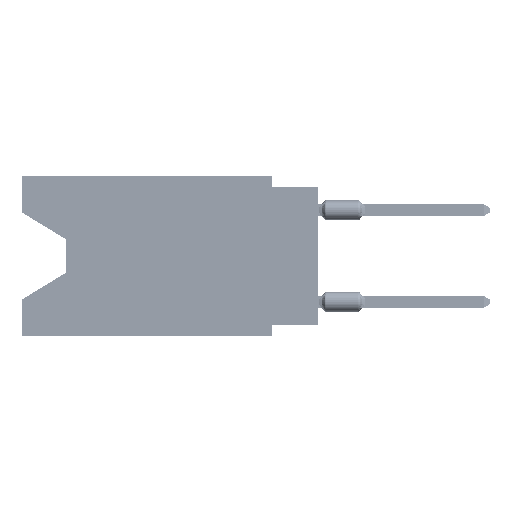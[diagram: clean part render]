
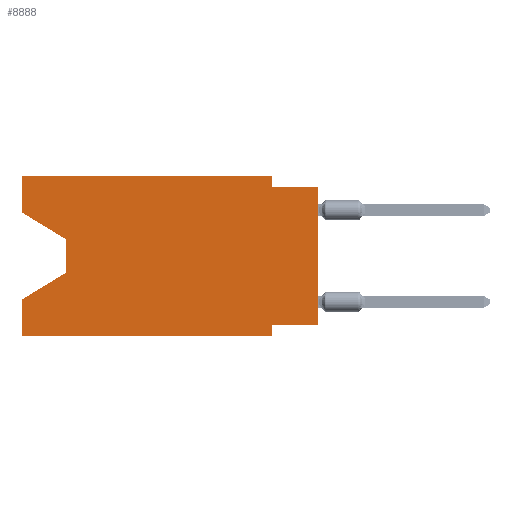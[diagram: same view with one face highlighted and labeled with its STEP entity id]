
A CAD part, left-side view. The second image highlights one B-rep face of the part: STEP entity #8888.
In plain terms, the highlighted planar face has unit normal (-1, 0, 0).
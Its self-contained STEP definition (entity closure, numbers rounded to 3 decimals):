
#288 = LINE ( 'NONE', #77231, #19993 ) ;
#1683 = LINE ( 'NONE', #27493, #95369 ) ;
#2556 = DIRECTION ( 'NONE',  ( 0., 0., -1. ) ) ;
#2775 = FACE_OUTER_BOUND ( 'NONE', #65414, .T. ) ;
#5400 = LINE ( 'NONE', #40770, #51607 ) ;
#8888 = ADVANCED_FACE ( 'NONE', ( #2775 ), #20752, .F. ) ;
#9208 = EDGE_CURVE ( 'NONE', #75606, #36875, #27916, .T. ) ;
#9214 = ORIENTED_EDGE ( 'NONE', *, *, #74387, .F. ) ;
#10415 = LINE ( 'NONE', #87878, #76460 ) ;
#10650 = DIRECTION ( 'NONE',  ( 0., 0.855, -0.519 ) ) ;
#13079 = ORIENTED_EDGE ( 'NONE', *, *, #45619, .F. ) ;
#13785 = EDGE_CURVE ( 'NONE', #82977, #32922, #1683, .T. ) ;
#15249 = VERTEX_POINT ( 'NONE', #76279 ) ;
#15433 = VECTOR ( 'NONE', #10650, 1000. ) ;
#15911 = LINE ( 'NONE', #50157, #105549 ) ;
#19244 = EDGE_CURVE ( 'NONE', #72556, #80418, #110894, .T. ) ;
#19993 = VECTOR ( 'NONE', #67709, 1000. ) ;
#20187 = DIRECTION ( 'NONE',  ( 0., 0., -1. ) ) ;
#20752 = PLANE ( 'NONE',  #31515 ) ;
#20849 = CARTESIAN_POINT ( 'NONE',  ( 0., 2.54, -0.635 ) ) ;
#22002 = VERTEX_POINT ( 'NONE', #46269 ) ;
#25535 = ORIENTED_EDGE ( 'NONE', *, *, #9208, .T. ) ;
#25588 = DIRECTION ( 'NONE',  ( 0., 0., 1. ) ) ;
#27133 = EDGE_CURVE ( 'NONE', #72268, #80418, #10415, .T. ) ;
#27493 = CARTESIAN_POINT ( 'NONE',  ( 0., 16.383, 0. ) ) ;
#27916 = LINE ( 'NONE', #103693, #65675 ) ;
#28185 = VECTOR ( 'NONE', #76021, 1000. ) ;
#28378 = DIRECTION ( 'NONE',  ( 0., -1., 0. ) ) ;
#29636 = EDGE_CURVE ( 'NONE', #94697, #36875, #5400, .T. ) ;
#30565 = CARTESIAN_POINT ( 'NONE',  ( 0., 16.383, -6.852 ) ) ;
#31515 = AXIS2_PLACEMENT_3D ( 'NONE', #78600, #70171, #20187 ) ;
#32922 = VERTEX_POINT ( 'NONE', #55768 ) ;
#34247 = CARTESIAN_POINT ( 'NONE',  ( 0., 2.54, -8.89 ) ) ;
#35544 = EDGE_CURVE ( 'NONE', #72556, #94697, #288, .T. ) ;
#36875 = VERTEX_POINT ( 'NONE', #34247 ) ;
#37188 = VECTOR ( 'NONE', #2556, 1000. ) ;
#40404 = ORIENTED_EDGE ( 'NONE', *, *, #53197, .T. ) ;
#40538 = CARTESIAN_POINT ( 'NONE',  ( 0., 16.383, -2.038 ) ) ;
#40770 = CARTESIAN_POINT ( 'NONE',  ( 0., 2.54, -8.89 ) ) ;
#45619 = EDGE_CURVE ( 'NONE', #32922, #72268, #87361, .T. ) ;
#46269 = CARTESIAN_POINT ( 'NONE',  ( 0., 13.97, -3.505 ) ) ;
#47875 = EDGE_CURVE ( 'NONE', #22002, #15249, #76580, .T. ) ;
#48925 = CARTESIAN_POINT ( 'NONE',  ( 0., 16.383, 0. ) ) ;
#50157 = CARTESIAN_POINT ( 'NONE',  ( 0., 16.383, -2.038 ) ) ;
#51004 = VECTOR ( 'NONE', #84812, 1000. ) ;
#51607 = VECTOR ( 'NONE', #64923, 1000. ) ;
#51693 = EDGE_CURVE ( 'NONE', #56180, #22002, #15911, .T. ) ;
#51742 = ORIENTED_EDGE ( 'NONE', *, *, #29636, .F. ) ;
#53197 = EDGE_CURVE ( 'NONE', #15249, #55713, #61727, .T. ) ;
#53533 = CARTESIAN_POINT ( 'NONE',  ( 0., 2.54, -8.255 ) ) ;
#54604 = ORIENTED_EDGE ( 'NONE', *, *, #35544, .F. ) ;
#55713 = VERTEX_POINT ( 'NONE', #30565 ) ;
#55768 = CARTESIAN_POINT ( 'NONE',  ( 0., 2.54, 0. ) ) ;
#56180 = VERTEX_POINT ( 'NONE', #40538 ) ;
#56552 = CARTESIAN_POINT ( 'NONE',  ( 0., 16.383, -8.89 ) ) ;
#57354 = LINE ( 'NONE', #48925, #51004 ) ;
#57825 = VECTOR ( 'NONE', #73945, 1000. ) ;
#61727 = LINE ( 'NONE', #94857, #15433 ) ;
#64923 = DIRECTION ( 'NONE',  ( 0., 0., -1. ) ) ;
#65414 = EDGE_LOOP ( 'NONE', ( #109851, #103814, #40404, #68416, #25535, #51742, #54604, #96321, #89580, #13079, #77103, #9214 ) ) ;
#65524 = LINE ( 'NONE', #67177, #57825 ) ;
#65675 = VECTOR ( 'NONE', #95823, 1000. ) ;
#67177 = CARTESIAN_POINT ( 'NONE',  ( 0., 16.383, 0. ) ) ;
#67709 = DIRECTION ( 'NONE',  ( 0., 1., 0. ) ) ;
#68416 = ORIENTED_EDGE ( 'NONE', *, *, #101484, .F. ) ;
#70171 = DIRECTION ( 'NONE',  ( 1., 0., 0. ) ) ;
#72268 = VERTEX_POINT ( 'NONE', #20849 ) ;
#72556 = VERTEX_POINT ( 'NONE', #89258 ) ;
#73945 = DIRECTION ( 'NONE',  ( 0., 0., 1. ) ) ;
#74387 = EDGE_CURVE ( 'NONE', #56180, #82977, #65524, .T. ) ;
#75606 = VERTEX_POINT ( 'NONE', #56552 ) ;
#76021 = DIRECTION ( 'NONE',  ( 0., 0., -1. ) ) ;
#76279 = CARTESIAN_POINT ( 'NONE',  ( 0., 13.97, -5.385 ) ) ;
#76460 = VECTOR ( 'NONE', #28378, 1000. ) ;
#76580 = LINE ( 'NONE', #84437, #28185 ) ;
#77103 = ORIENTED_EDGE ( 'NONE', *, *, #13785, .F. ) ;
#77231 = CARTESIAN_POINT ( 'NONE',  ( 0., 0., -8.255 ) ) ;
#78600 = CARTESIAN_POINT ( 'NONE',  ( 0., 16.383, 0. ) ) ;
#80418 = VERTEX_POINT ( 'NONE', #100712 ) ;
#81843 = VECTOR ( 'NONE', #25588, 1000. ) ;
#82977 = VERTEX_POINT ( 'NONE', #95128 ) ;
#84388 = DIRECTION ( 'NONE',  ( 0., -0.855, -0.519 ) ) ;
#84437 = CARTESIAN_POINT ( 'NONE',  ( 0., 13.97, -3.505 ) ) ;
#84812 = DIRECTION ( 'NONE',  ( 0., 0., 1. ) ) ;
#87361 = LINE ( 'NONE', #106356, #37188 ) ;
#87878 = CARTESIAN_POINT ( 'NONE',  ( 0., 0., -0.635 ) ) ;
#89258 = CARTESIAN_POINT ( 'NONE',  ( 0., 0., -8.255 ) ) ;
#89580 = ORIENTED_EDGE ( 'NONE', *, *, #27133, .F. ) ;
#94697 = VERTEX_POINT ( 'NONE', #53533 ) ;
#94857 = CARTESIAN_POINT ( 'NONE',  ( 0., 13.97, -5.385 ) ) ;
#95128 = CARTESIAN_POINT ( 'NONE',  ( 0., 16.383, 0. ) ) ;
#95369 = VECTOR ( 'NONE', #95964, 1000. ) ;
#95823 = DIRECTION ( 'NONE',  ( 0., -1., 0. ) ) ;
#95964 = DIRECTION ( 'NONE',  ( 0., -1., 0. ) ) ;
#96321 = ORIENTED_EDGE ( 'NONE', *, *, #19244, .T. ) ;
#100712 = CARTESIAN_POINT ( 'NONE',  ( 0., 0., -0.635 ) ) ;
#101484 = EDGE_CURVE ( 'NONE', #75606, #55713, #57354, .T. ) ;
#102459 = CARTESIAN_POINT ( 'NONE',  ( 0., 0., 0. ) ) ;
#103693 = CARTESIAN_POINT ( 'NONE',  ( 0., 16.383, -8.89 ) ) ;
#103814 = ORIENTED_EDGE ( 'NONE', *, *, #47875, .T. ) ;
#105549 = VECTOR ( 'NONE', #84388, 1000. ) ;
#106356 = CARTESIAN_POINT ( 'NONE',  ( 0., 2.54, 0. ) ) ;
#109851 = ORIENTED_EDGE ( 'NONE', *, *, #51693, .T. ) ;
#110894 = LINE ( 'NONE', #102459, #81843 ) ;
